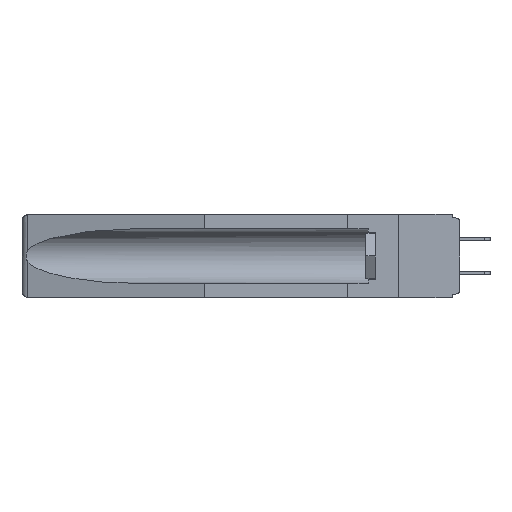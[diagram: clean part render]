
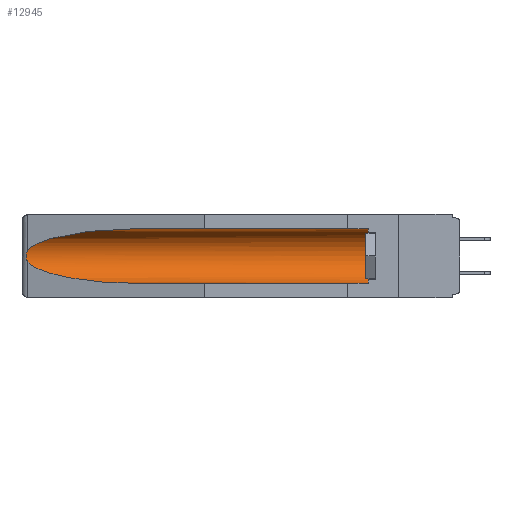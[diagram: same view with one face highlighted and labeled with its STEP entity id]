
A CAD part, left-side view. The second image highlights one B-rep face of the part: STEP entity #12945.
In plain terms, the highlighted cylindrical face has radius 2.857 mm (diameter 5.715 mm), a partial arc.
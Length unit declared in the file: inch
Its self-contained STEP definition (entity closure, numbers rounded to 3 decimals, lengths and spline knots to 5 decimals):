
#100 = VECTOR ( 'NONE', #18753, 39.37008 ) ;
#160 = CARTESIAN_POINT ( 'NONE',  ( 0.26655, 1.53094, -0.18657 ) ) ;
#767 = ORIENTED_EDGE ( 'NONE', *, *, #10673, .T. ) ;
#1196 = FACE_OUTER_BOUND ( 'NONE', #11339, .T. ) ;
#1204 = EDGE_CURVE ( 'NONE', #15650, #5337, #15448, .T. ) ;
#1860 = EDGE_CURVE ( 'NONE', #5118, #3221, #7377, .T. ) ;
#2030 = EDGE_CURVE ( 'NONE', #18578, #3221, #4140, .T. ) ;
#2168 = CARTESIAN_POINT ( 'NONE',  ( 0.155, 1.07973, -0.059 ) ) ;
#2184 = VECTOR ( 'NONE', #6545, 39.37008 ) ;
#2593 = CARTESIAN_POINT ( 'NONE',  ( 0.155, 0.126, -0.284 ) ) ;
#3145 = CARTESIAN_POINT ( 'NONE',  ( 0.2675, 1.53308, -0.16763 ) ) ;
#3212 = CARTESIAN_POINT ( 'NONE',  ( 0.26537, 1.52718, -0.19328 ) ) ;
#3221 = VERTEX_POINT ( 'NONE', #11774 ) ;
#3581 = CARTESIAN_POINT ( 'NONE',  ( 0.155, -0.30754, -0.059 ) ) ;
#3634 = CYLINDRICAL_SURFACE ( 'NONE', #15281, 0.1125 ) ;
#4037 = ORIENTED_EDGE ( 'NONE', *, *, #1204, .T. ) ;
#4140 = LINE ( 'NONE', #4844, #100 ) ;
#4286 = CARTESIAN_POINT ( 'NONE',  ( 0.155, -0.30754, -0.1715 ) ) ;
#4844 = CARTESIAN_POINT ( 'NONE',  ( 0.155, -0.30754, -0.284 ) ) ;
#4923 = B_SPLINE_CURVE_WITH_KNOTS ( 'NONE', 3,
 ( #12407, #15506, #7727, #18530, #3145, #6215, #17040, #160, #12469, #3212 ),
 .UNSPECIFIED., .F., .F.,
 ( 4, 2, 2, 2, 4 ),
 ( 0., 0.00029, 0.00058, 0.00087, 0.00117 ),
 .UNSPECIFIED. ) ;
#5118 = VERTEX_POINT ( 'NONE', #15120 ) ;
#5337 = VERTEX_POINT ( 'NONE', #17577 ) ;
#5447 = CARTESIAN_POINT ( 'NONE',  ( 0.25451, 1.48313, -0.24835 ) ) ;
#5706 = DIRECTION ( 'NONE',  ( 0., 0., 1. ) ) ;
#6215 = CARTESIAN_POINT ( 'NONE',  ( 0.2675, 1.53308, -0.17534 ) ) ;
#6545 = DIRECTION ( 'NONE',  ( 0., 1., 0. ) ) ;
#7006 = CARTESIAN_POINT ( 'NONE',  ( 0.21114, 1.30732, -0.284 ) ) ;
#7377 =( BOUNDED_CURVE ( )  B_SPLINE_CURVE ( 3, ( #19653, #5447, #7006, #12428 ),
 .UNSPECIFIED., .F., .F. ) 
 B_SPLINE_CURVE_WITH_KNOTS ( ( 4, 4 ),
 ( 0.1948, 1.5708 ),
 .UNSPECIFIED. ) 
 CURVE ( )  GEOMETRIC_REPRESENTATION_ITEM ( )  RATIONAL_B_SPLINE_CURVE ( ( 1., 0.848, 0.848, 1. ) ) 
 REPRESENTATION_ITEM ( '' )  );
#7464 = ORIENTED_EDGE ( 'NONE', *, *, #1860, .T. ) ;
#7727 = CARTESIAN_POINT ( 'NONE',  ( 0.26654, 1.53092, -0.15636 ) ) ;
#8020 = CARTESIAN_POINT ( 'NONE',  ( 0.25451, 1.48313, -0.09465 ) ) ;
#8350 = DIRECTION ( 'NONE',  ( 0., -1., 0. ) ) ;
#9013 = ORIENTED_EDGE ( 'NONE', *, *, #2030, .F. ) ;
#10673 = EDGE_CURVE ( 'NONE', #5337, #5118, #4923, .T. ) ;
#10708 = VERTEX_POINT ( 'NONE', #12733 ) ;
#10814 = CARTESIAN_POINT ( 'NONE',  ( 0.26537, 1.52718, -0.14972 ) ) ;
#11339 = EDGE_LOOP ( 'NONE', ( #4037, #767, #7464, #9013, #19173, #11932 ) ) ;
#11774 = CARTESIAN_POINT ( 'NONE',  ( 0.155, 1.07973, -0.284 ) ) ;
#11932 = ORIENTED_EDGE ( 'NONE', *, *, #16701, .T. ) ;
#12407 = CARTESIAN_POINT ( 'NONE',  ( 0.26537, 1.52718, -0.14972 ) ) ;
#12428 = CARTESIAN_POINT ( 'NONE',  ( 0.155, 1.07973, -0.284 ) ) ;
#12469 = CARTESIAN_POINT ( 'NONE',  ( 0.26597, 1.5296, -0.19026 ) ) ;
#12719 = EDGE_CURVE ( 'NONE', #18578, #10708, #17492, .T. ) ;
#12733 = CARTESIAN_POINT ( 'NONE',  ( 0.155, 0.126, -0.059 ) ) ;
#12945 = ADVANCED_FACE ( 'NONE', ( #1196 ), #3634, .F. ) ;
#14719 = LINE ( 'NONE', #3581, #2184 ) ;
#15120 = CARTESIAN_POINT ( 'NONE',  ( 0.26537, 1.52718, -0.19328 ) ) ;
#15281 = AXIS2_PLACEMENT_3D ( 'NONE', #4286, #18122, #5706 ) ;
#15448 =( BOUNDED_CURVE ( )  B_SPLINE_CURVE ( 3, ( #18693, #17205, #8020, #10814 ),
 .UNSPECIFIED., .F., .F. ) 
 B_SPLINE_CURVE_WITH_KNOTS ( ( 4, 4 ),
 ( 4.71239, 6.08839 ),
 .UNSPECIFIED. ) 
 CURVE ( )  GEOMETRIC_REPRESENTATION_ITEM ( )  RATIONAL_B_SPLINE_CURVE ( ( 1., 0.848, 0.848, 1. ) ) 
 REPRESENTATION_ITEM ( '' )  );
#15506 = CARTESIAN_POINT ( 'NONE',  ( 0.26597, 1.52961, -0.15275 ) ) ;
#15645 = AXIS2_PLACEMENT_3D ( 'NONE', #16112, #8350, #19154 ) ;
#15650 = VERTEX_POINT ( 'NONE', #2168 ) ;
#16112 = CARTESIAN_POINT ( 'NONE',  ( 0.155, 0.126, -0.1715 ) ) ;
#16701 = EDGE_CURVE ( 'NONE', #10708, #15650, #14719, .T. ) ;
#17040 = CARTESIAN_POINT ( 'NONE',  ( 0.2673, 1.53269, -0.17917 ) ) ;
#17205 = CARTESIAN_POINT ( 'NONE',  ( 0.21114, 1.30732, -0.059 ) ) ;
#17492 = CIRCLE ( 'NONE', #15645, 0.1125 ) ;
#17577 = CARTESIAN_POINT ( 'NONE',  ( 0.26537, 1.52718, -0.14972 ) ) ;
#18122 = DIRECTION ( 'NONE',  ( 0., 1., 0. ) ) ;
#18530 = CARTESIAN_POINT ( 'NONE',  ( 0.2673, 1.5327, -0.16383 ) ) ;
#18578 = VERTEX_POINT ( 'NONE', #2593 ) ;
#18693 = CARTESIAN_POINT ( 'NONE',  ( 0.155, 1.07973, -0.059 ) ) ;
#18753 = DIRECTION ( 'NONE',  ( 0., 1., 0. ) ) ;
#19154 = DIRECTION ( 'NONE',  ( 0., 0., 1. ) ) ;
#19173 = ORIENTED_EDGE ( 'NONE', *, *, #12719, .T. ) ;
#19653 = CARTESIAN_POINT ( 'NONE',  ( 0.26537, 1.52718, -0.19328 ) ) ;
